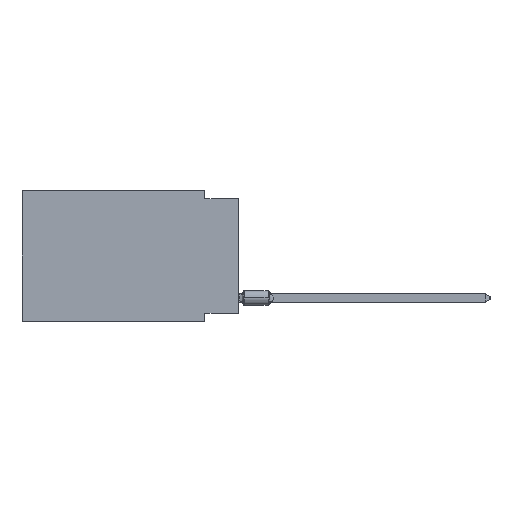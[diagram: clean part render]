
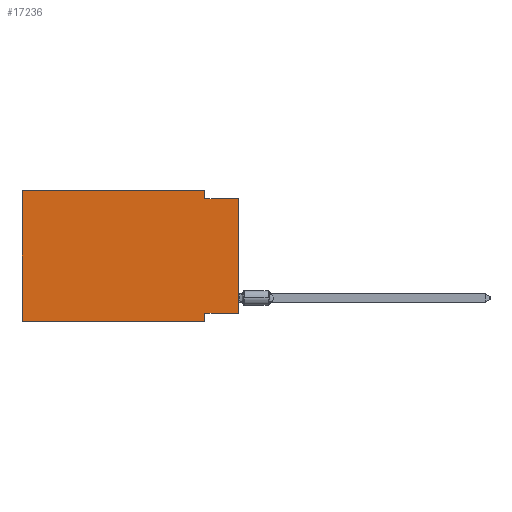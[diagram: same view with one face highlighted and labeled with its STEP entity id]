
A CAD part, left-side view. The second image highlights one B-rep face of the part: STEP entity #17236.
In plain terms, the highlighted planar face has unit normal (-1, 0, 0).
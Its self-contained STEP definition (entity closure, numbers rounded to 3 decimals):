
#46 = VERTEX_POINT ( 'NONE', #37012 ) ;
#93 = VECTOR ( 'NONE', #35018, 1000. ) ;
#1046 = ORIENTED_EDGE ( 'NONE', *, *, #23285, .F. ) ;
#1510 = AXIS2_PLACEMENT_3D ( 'NONE', #15381, #29555, #31822 ) ;
#1644 = CARTESIAN_POINT ( 'NONE',  ( 0., 16.383, -9.906 ) ) ;
#2520 = LINE ( 'NONE', #14077, #15607 ) ;
#2962 = DIRECTION ( 'NONE',  ( 0., -1., 0. ) ) ;
#3468 = CARTESIAN_POINT ( 'NONE',  ( 0., 2.54, -9.906 ) ) ;
#4738 = CARTESIAN_POINT ( 'NONE',  ( 0., 0., 0. ) ) ;
#6060 = EDGE_LOOP ( 'NONE', ( #24222, #35022, #29696, #20544, #7946, #23560, #32012, #1046 ) ) ;
#6103 = CARTESIAN_POINT ( 'NONE',  ( 0., 2.54, -9.271 ) ) ;
#6205 = VERTEX_POINT ( 'NONE', #29363 ) ;
#7156 = DIRECTION ( 'NONE',  ( 0., 0., 1. ) ) ;
#7908 = VERTEX_POINT ( 'NONE', #32252 ) ;
#7946 = ORIENTED_EDGE ( 'NONE', *, *, #36906, .F. ) ;
#9556 = DIRECTION ( 'NONE',  ( 0., 0., 1. ) ) ;
#12171 = LINE ( 'NONE', #3468, #22861 ) ;
#12225 = VECTOR ( 'NONE', #7156, 1000. ) ;
#12370 = EDGE_CURVE ( 'NONE', #33708, #16632, #18710, .T. ) ;
#12660 = VECTOR ( 'NONE', #2962, 1000. ) ;
#14077 = CARTESIAN_POINT ( 'NONE',  ( 0., 2.54, 0. ) ) ;
#14243 = EDGE_CURVE ( 'NONE', #19070, #46, #35271, .T. ) ;
#15381 = CARTESIAN_POINT ( 'NONE',  ( 0., 16.383, 0. ) ) ;
#15607 = VECTOR ( 'NONE', #25603, 1000. ) ;
#16632 = VERTEX_POINT ( 'NONE', #22980 ) ;
#17014 = DIRECTION ( 'NONE',  ( 0., 1., 0. ) ) ;
#17236 = ADVANCED_FACE ( 'NONE', ( #20482 ), #26912, .F. ) ;
#18710 = LINE ( 'NONE', #1644, #33259 ) ;
#19070 = VERTEX_POINT ( 'NONE', #36416 ) ;
#19590 = VECTOR ( 'NONE', #17014, 1000. ) ;
#19666 = LINE ( 'NONE', #34229, #19590 ) ;
#20183 = CARTESIAN_POINT ( 'NONE',  ( 0., 16.383, 0. ) ) ;
#20482 = FACE_OUTER_BOUND ( 'NONE', #6060, .T. ) ;
#20544 = ORIENTED_EDGE ( 'NONE', *, *, #21790, .F. ) ;
#20642 = LINE ( 'NONE', #26518, #93 ) ;
#21790 = EDGE_CURVE ( 'NONE', #6205, #32667, #25277, .T. ) ;
#22861 = VECTOR ( 'NONE', #23881, 1000. ) ;
#22980 = CARTESIAN_POINT ( 'NONE',  ( 0., 2.54, -9.906 ) ) ;
#23285 = EDGE_CURVE ( 'NONE', #19070, #28844, #19666, .T. ) ;
#23560 = ORIENTED_EDGE ( 'NONE', *, *, #12370, .T. ) ;
#23881 = DIRECTION ( 'NONE',  ( 0., 0., -1. ) ) ;
#24222 = ORIENTED_EDGE ( 'NONE', *, *, #14243, .T. ) ;
#24923 = DIRECTION ( 'NONE',  ( 0., -1., 0. ) ) ;
#25277 = LINE ( 'NONE', #20183, #12660 ) ;
#25603 = DIRECTION ( 'NONE',  ( 0., 0., -1. ) ) ;
#26518 = CARTESIAN_POINT ( 'NONE',  ( 0., 0., -0.635 ) ) ;
#26912 = PLANE ( 'NONE',  #1510 ) ;
#28083 = CARTESIAN_POINT ( 'NONE',  ( 0., 2.54, 0. ) ) ;
#28844 = VERTEX_POINT ( 'NONE', #6103 ) ;
#29363 = CARTESIAN_POINT ( 'NONE',  ( 0., 16.383, 0. ) ) ;
#29555 = DIRECTION ( 'NONE',  ( 1., 0., 0. ) ) ;
#29696 = ORIENTED_EDGE ( 'NONE', *, *, #30444, .F. ) ;
#30444 = EDGE_CURVE ( 'NONE', #32667, #7908, #2520, .T. ) ;
#30578 = LINE ( 'NONE', #32696, #12225 ) ;
#30600 = EDGE_CURVE ( 'NONE', #28844, #16632, #12171, .T. ) ;
#31822 = DIRECTION ( 'NONE',  ( 0., 0., -1. ) ) ;
#32012 = ORIENTED_EDGE ( 'NONE', *, *, #30600, .F. ) ;
#32252 = CARTESIAN_POINT ( 'NONE',  ( 0., 2.54, -0.635 ) ) ;
#32548 = CARTESIAN_POINT ( 'NONE',  ( 0., 16.383, -9.906 ) ) ;
#32667 = VERTEX_POINT ( 'NONE', #28083 ) ;
#32696 = CARTESIAN_POINT ( 'NONE',  ( 0., 16.383, 0. ) ) ;
#33259 = VECTOR ( 'NONE', #24923, 1000. ) ;
#33708 = VERTEX_POINT ( 'NONE', #32548 ) ;
#34229 = CARTESIAN_POINT ( 'NONE',  ( 0., 0., -9.271 ) ) ;
#34619 = EDGE_CURVE ( 'NONE', #7908, #46, #20642, .T. ) ;
#35018 = DIRECTION ( 'NONE',  ( 0., -1., 0. ) ) ;
#35022 = ORIENTED_EDGE ( 'NONE', *, *, #34619, .F. ) ;
#35271 = LINE ( 'NONE', #4738, #37034 ) ;
#36416 = CARTESIAN_POINT ( 'NONE',  ( 0., 0., -9.271 ) ) ;
#36906 = EDGE_CURVE ( 'NONE', #33708, #6205, #30578, .T. ) ;
#37012 = CARTESIAN_POINT ( 'NONE',  ( 0., 0., -0.635 ) ) ;
#37034 = VECTOR ( 'NONE', #9556, 1000. ) ;
